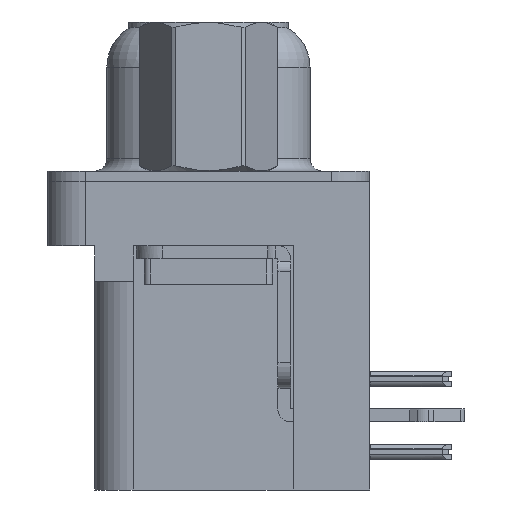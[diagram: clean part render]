
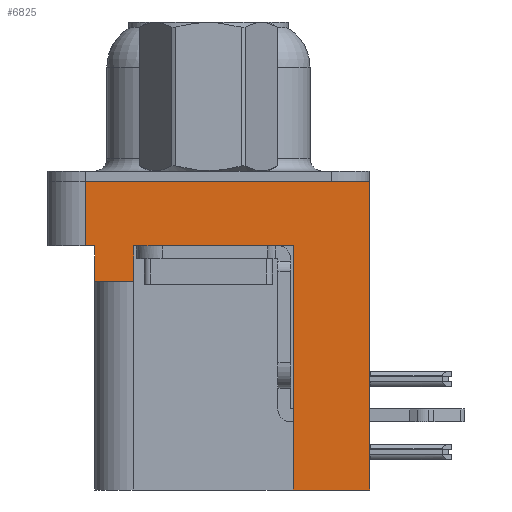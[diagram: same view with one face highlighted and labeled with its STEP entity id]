
A CAD part, left-side view. The second image highlights one B-rep face of the part: STEP entity #6825.
In plain terms, the highlighted planar face has unit normal (-1, 0, 0).
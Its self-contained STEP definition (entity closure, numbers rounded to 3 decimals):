
#1276 = VECTOR ( 'NONE', #11965, 1000. ) ;
#1792 = DIRECTION ( 'NONE',  ( 0., -1., 0. ) ) ;
#1973 = VECTOR ( 'NONE', #34666, 1000. ) ;
#2191 = LINE ( 'NONE', #15132, #33429 ) ;
#2270 = CARTESIAN_POINT ( 'NONE',  ( -3., 4.425, -3.9 ) ) ;
#2922 = EDGE_CURVE ( 'NONE', #33286, #27407, #25095, .T. ) ;
#3086 = EDGE_CURVE ( 'NONE', #24420, #4154, #12072, .T. ) ;
#3331 = CARTESIAN_POINT ( 'NONE',  ( -3., -6.275, -2.5 ) ) ;
#3709 = CARTESIAN_POINT ( 'NONE',  ( -3., 4.425, -2.5 ) ) ;
#3850 = DIRECTION ( 'NONE',  ( 0., 0., 1. ) ) ;
#3857 = CARTESIAN_POINT ( 'NONE',  ( -3., -6.275, -12. ) ) ;
#3881 = CARTESIAN_POINT ( 'NONE',  ( -3., -3.295, -12. ) ) ;
#4154 = VERTEX_POINT ( 'NONE', #3709 ) ;
#4928 = CARTESIAN_POINT ( 'NONE',  ( -3., 2.895, -2.5 ) ) ;
#4933 = LINE ( 'NONE', #10069, #12723 ) ;
#5562 = CARTESIAN_POINT ( 'NONE',  ( -3., -6.275, 0. ) ) ;
#5927 = ORIENTED_EDGE ( 'NONE', *, *, #25658, .T. ) ;
#5946 = ORIENTED_EDGE ( 'NONE', *, *, #29186, .F. ) ;
#6071 = DIRECTION ( 'NONE',  ( 0., -1., 0. ) ) ;
#6372 = EDGE_LOOP ( 'NONE', ( #5946, #31087, #14644, #10386, #30342, #30464, #5927, #32747, #9448, #10668 ) ) ;
#6735 = CARTESIAN_POINT ( 'NONE',  ( -3., -3.295, -2.5 ) ) ;
#6825 = ADVANCED_FACE ( 'NONE', ( #14443 ), #22168, .T. ) ;
#6852 = VECTOR ( 'NONE', #32006, 1000. ) ;
#7497 = DIRECTION ( 'NONE',  ( 0., 1., 0. ) ) ;
#8328 = DIRECTION ( 'NONE',  ( 0., 0., 1. ) ) ;
#8595 = VERTEX_POINT ( 'NONE', #3881 ) ;
#9448 = ORIENTED_EDGE ( 'NONE', *, *, #33449, .F. ) ;
#9493 = LINE ( 'NONE', #3331, #29941 ) ;
#10069 = CARTESIAN_POINT ( 'NONE',  ( -3., -3.295, -12. ) ) ;
#10386 = ORIENTED_EDGE ( 'NONE', *, *, #3086, .F. ) ;
#10668 = ORIENTED_EDGE ( 'NONE', *, *, #18438, .T. ) ;
#11678 = EDGE_CURVE ( 'NONE', #8595, #31245, #32947, .T. ) ;
#11965 = DIRECTION ( 'NONE',  ( 0., 0., 1. ) ) ;
#12072 = LINE ( 'NONE', #2270, #16848 ) ;
#12082 = LINE ( 'NONE', #32246, #6852 ) ;
#12585 = CARTESIAN_POINT ( 'NONE',  ( -3., 4.425, -3.9 ) ) ;
#12644 = CARTESIAN_POINT ( 'NONE',  ( -3., -6.275, 0. ) ) ;
#12718 = DIRECTION ( 'NONE',  ( 0., -1., 0. ) ) ;
#12723 = VECTOR ( 'NONE', #7497, 1000. ) ;
#12807 = DIRECTION ( 'NONE',  ( 0., 0., 1. ) ) ;
#12860 = VERTEX_POINT ( 'NONE', #3857 ) ;
#14003 = DIRECTION ( 'NONE',  ( -1., 0., 0. ) ) ;
#14091 = AXIS2_PLACEMENT_3D ( 'NONE', #27651, #14003, #8328 ) ;
#14300 = VECTOR ( 'NONE', #12807, 1000. ) ;
#14443 = FACE_OUTER_BOUND ( 'NONE', #6372, .T. ) ;
#14621 = EDGE_CURVE ( 'NONE', #27188, #25577, #22329, .T. ) ;
#14644 = ORIENTED_EDGE ( 'NONE', *, *, #34942, .T. ) ;
#14926 = VECTOR ( 'NONE', #1792, 1000. ) ;
#15132 = CARTESIAN_POINT ( 'NONE',  ( -3., -6.275, -2.5 ) ) ;
#15436 = CARTESIAN_POINT ( 'NONE',  ( -3., 4.775, -2.5 ) ) ;
#16565 = VERTEX_POINT ( 'NONE', #5562 ) ;
#16848 = VECTOR ( 'NONE', #27198, 1000. ) ;
#18438 = EDGE_CURVE ( 'NONE', #12860, #16565, #29986, .T. ) ;
#20477 = CARTESIAN_POINT ( 'NONE',  ( -3., 4.775, 0. ) ) ;
#20712 = VECTOR ( 'NONE', #3850, 1000. ) ;
#20774 = CARTESIAN_POINT ( 'NONE',  ( -3., 2.895, -3.9 ) ) ;
#20948 = EDGE_CURVE ( 'NONE', #33286, #24420, #12082, .T. ) ;
#21041 = CARTESIAN_POINT ( 'NONE',  ( -3., -6.275, -2.5 ) ) ;
#21442 = LINE ( 'NONE', #12644, #14926 ) ;
#22168 = PLANE ( 'NONE',  #14091 ) ;
#22329 = LINE ( 'NONE', #15436, #1973 ) ;
#24420 = VERTEX_POINT ( 'NONE', #12585 ) ;
#25095 = LINE ( 'NONE', #20774, #1276 ) ;
#25269 = CARTESIAN_POINT ( 'NONE',  ( -3., -3.295, -12. ) ) ;
#25577 = VERTEX_POINT ( 'NONE', #20477 ) ;
#25658 = EDGE_CURVE ( 'NONE', #27407, #31245, #2191, .T. ) ;
#27188 = VERTEX_POINT ( 'NONE', #33236 ) ;
#27198 = DIRECTION ( 'NONE',  ( 0., 0., 1. ) ) ;
#27407 = VERTEX_POINT ( 'NONE', #4928 ) ;
#27651 = CARTESIAN_POINT ( 'NONE',  ( -3., -6.275, -2.5 ) ) ;
#29161 = CARTESIAN_POINT ( 'NONE',  ( -3., 2.895, -3.9 ) ) ;
#29186 = EDGE_CURVE ( 'NONE', #25577, #16565, #21442, .T. ) ;
#29941 = VECTOR ( 'NONE', #6071, 1000. ) ;
#29986 = LINE ( 'NONE', #21041, #14300 ) ;
#30342 = ORIENTED_EDGE ( 'NONE', *, *, #20948, .F. ) ;
#30464 = ORIENTED_EDGE ( 'NONE', *, *, #2922, .T. ) ;
#31087 = ORIENTED_EDGE ( 'NONE', *, *, #14621, .F. ) ;
#31245 = VERTEX_POINT ( 'NONE', #6735 ) ;
#32006 = DIRECTION ( 'NONE',  ( 0., 1., 0. ) ) ;
#32246 = CARTESIAN_POINT ( 'NONE',  ( -3., 4.425, -3.9 ) ) ;
#32747 = ORIENTED_EDGE ( 'NONE', *, *, #11678, .F. ) ;
#32947 = LINE ( 'NONE', #25269, #20712 ) ;
#33236 = CARTESIAN_POINT ( 'NONE',  ( -3., 4.775, -2.5 ) ) ;
#33286 = VERTEX_POINT ( 'NONE', #29161 ) ;
#33429 = VECTOR ( 'NONE', #12718, 1000. ) ;
#33449 = EDGE_CURVE ( 'NONE', #12860, #8595, #4933, .T. ) ;
#34666 = DIRECTION ( 'NONE',  ( 0., 0., 1. ) ) ;
#34942 = EDGE_CURVE ( 'NONE', #27188, #4154, #9493, .T. ) ;
